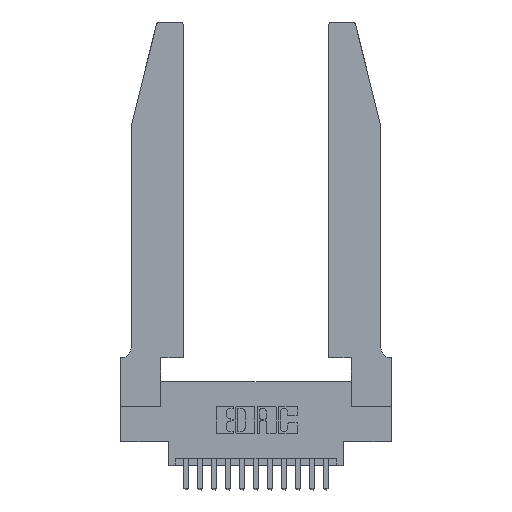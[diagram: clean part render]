
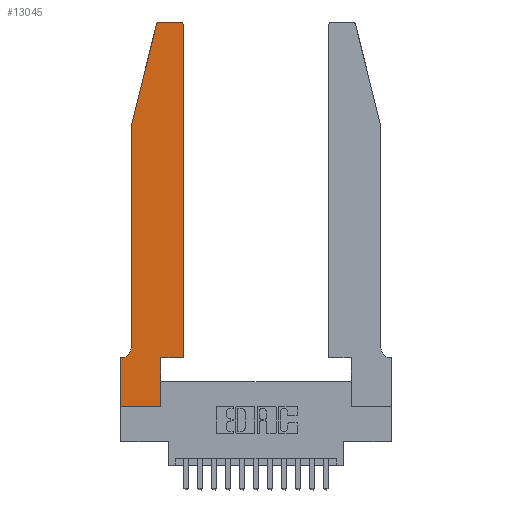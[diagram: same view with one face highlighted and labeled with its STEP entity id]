
A CAD part, top view. The second image highlights one B-rep face of the part: STEP entity #13045.
In plain terms, the highlighted planar face has unit normal (0, 0, 1).
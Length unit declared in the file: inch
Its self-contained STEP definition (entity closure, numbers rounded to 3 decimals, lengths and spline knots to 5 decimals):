
#377 = CARTESIAN_POINT ( 'NONE',  ( 0.0055, 0.35, 0.37 ) ) ;
#400 = EDGE_CURVE ( 'NONE', #11170, #15418, #11970, .T. ) ;
#570 = DIRECTION ( 'NONE',  ( 0., 0., -1. ) ) ;
#1208 = CARTESIAN_POINT ( 'NONE',  ( 0.0755, 0.35, 0.37 ) ) ;
#1275 = EDGE_LOOP ( 'NONE', ( #4739, #13195, #8741, #8817, #12159, #3597, #8021, #15969, #4738, #7466, #9636, #4335 ) ) ;
#1544 = VERTEX_POINT ( 'NONE', #4493 ) ;
#1551 = CIRCLE ( 'NONE', #7059, 0.03 ) ;
#1685 = LINE ( 'NONE', #3859, #11786 ) ;
#1721 = CARTESIAN_POINT ( 'NONE',  ( 0.4505, 2.72, 0.37 ) ) ;
#1910 = LINE ( 'NONE', #7632, #5176 ) ;
#1978 = FACE_OUTER_BOUND ( 'NONE', #1275, .T. ) ;
#2134 = DIRECTION ( 'NONE',  ( -0.239, -0.971, 0. ) ) ;
#2139 = VERTEX_POINT ( 'NONE', #1721 ) ;
#2272 = VECTOR ( 'NONE', #16141, 39.37008 ) ;
#2835 = VERTEX_POINT ( 'NONE', #8503 ) ;
#2952 = DIRECTION ( 'NONE',  ( 0., -1., 0. ) ) ;
#3266 = CIRCLE ( 'NONE', #13099, 0.03 ) ;
#3464 = EDGE_CURVE ( 'NONE', #15039, #14809, #10603, .T. ) ;
#3597 = ORIENTED_EDGE ( 'NONE', *, *, #17119, .T. ) ;
#3839 = CARTESIAN_POINT ( 'NONE',  ( 0.284, 2.75, 0.37 ) ) ;
#3859 = CARTESIAN_POINT ( 'NONE',  ( 0.4505, 0.35, 0.37 ) ) ;
#4257 = AXIS2_PLACEMENT_3D ( 'NONE', #11421, #4598, #14184 ) ;
#4277 = VECTOR ( 'NONE', #15594, 39.37008 ) ;
#4335 = ORIENTED_EDGE ( 'NONE', *, *, #13483, .T. ) ;
#4493 = CARTESIAN_POINT ( 'NONE',  ( 0.25487, 2.72718, 0.37 ) ) ;
#4598 = DIRECTION ( 'NONE',  ( 0., 0., 1. ) ) ;
#4665 = EDGE_CURVE ( 'NONE', #2835, #5376, #10775, .T. ) ;
#4738 = ORIENTED_EDGE ( 'NONE', *, *, #400, .T. ) ;
#4739 = ORIENTED_EDGE ( 'NONE', *, *, #4665, .T. ) ;
#4741 = EDGE_CURVE ( 'NONE', #1544, #4983, #10352, .T. ) ;
#4758 = VERTEX_POINT ( 'NONE', #17173 ) ;
#4861 = CARTESIAN_POINT ( 'NONE',  ( 0.0755, 2., 0.37 ) ) ;
#4910 = DIRECTION ( 'NONE',  ( 0., 1., 0. ) ) ;
#4983 = VERTEX_POINT ( 'NONE', #9564 ) ;
#5176 = VECTOR ( 'NONE', #4910, 39.37008 ) ;
#5329 = CARTESIAN_POINT ( 'NONE',  ( 0.4205, 2.72, 0.37 ) ) ;
#5376 = VERTEX_POINT ( 'NONE', #3839 ) ;
#5891 = CARTESIAN_POINT ( 'NONE',  ( 0.2865, 0., 0.37 ) ) ;
#6089 = CARTESIAN_POINT ( 'NONE',  ( 0.2865, 0.35, 0.37 ) ) ;
#6273 = LINE ( 'NONE', #1208, #16716 ) ;
#6515 = EDGE_CURVE ( 'NONE', #15418, #10537, #1685, .T. ) ;
#6654 = CARTESIAN_POINT ( 'NONE',  ( 0.0755, 0.42, 0.37 ) ) ;
#6718 = DIRECTION ( 'NONE',  ( 1., 0., 0. ) ) ;
#6878 = DIRECTION ( 'NONE',  ( 0., 1., 0. ) ) ;
#7059 = AXIS2_PLACEMENT_3D ( 'NONE', #7509, #17018, #8874 ) ;
#7325 = VECTOR ( 'NONE', #2952, 39.37008 ) ;
#7466 = ORIENTED_EDGE ( 'NONE', *, *, #6515, .T. ) ;
#7509 = CARTESIAN_POINT ( 'NONE',  ( 0.284, 2.72, 0.37 ) ) ;
#7632 = CARTESIAN_POINT ( 'NONE',  ( 0.4505, 0.35, 0.37 ) ) ;
#8021 = ORIENTED_EDGE ( 'NONE', *, *, #9525, .T. ) ;
#8471 = CARTESIAN_POINT ( 'NONE',  ( 0.0755, 2., 0.37 ) ) ;
#8503 = CARTESIAN_POINT ( 'NONE',  ( 0.4205, 2.75, 0.37 ) ) ;
#8701 = PLANE ( 'NONE',  #4257 ) ;
#8741 = ORIENTED_EDGE ( 'NONE', *, *, #4741, .T. ) ;
#8817 = ORIENTED_EDGE ( 'NONE', *, *, #9351, .T. ) ;
#8874 = DIRECTION ( 'NONE',  ( 1., 0., 0. ) ) ;
#8885 = CARTESIAN_POINT ( 'NONE',  ( 0.0055, 0.42, 0.37 ) ) ;
#8993 = EDGE_CURVE ( 'NONE', #10537, #2139, #1910, .T. ) ;
#9351 = EDGE_CURVE ( 'NONE', #4983, #15039, #11357, .T. ) ;
#9525 = EDGE_CURVE ( 'NONE', #13062, #4758, #15203, .T. ) ;
#9564 = CARTESIAN_POINT ( 'NONE',  ( 0.0755, 2., 0.37 ) ) ;
#9636 = ORIENTED_EDGE ( 'NONE', *, *, #8993, .T. ) ;
#10256 = DIRECTION ( 'NONE',  ( -1., 0., 0. ) ) ;
#10352 = LINE ( 'NONE', #4861, #16721 ) ;
#10537 = VERTEX_POINT ( 'NONE', #13908 ) ;
#10603 = CIRCLE ( 'NONE', #11149, 0.07 ) ;
#10705 = DIRECTION ( 'NONE',  ( 1., 0., 0. ) ) ;
#10775 = LINE ( 'NONE', #11626, #13975 ) ;
#10837 = EDGE_CURVE ( 'NONE', #4758, #11170, #17282, .T. ) ;
#10852 = DIRECTION ( 'NONE',  ( -1., 0., 0. ) ) ;
#11149 = AXIS2_PLACEMENT_3D ( 'NONE', #8885, #570, #10256 ) ;
#11170 = VERTEX_POINT ( 'NONE', #5891 ) ;
#11357 = LINE ( 'NONE', #8471, #7325 ) ;
#11421 = CARTESIAN_POINT ( 'NONE',  ( 0., 0.35, 0.37 ) ) ;
#11626 = CARTESIAN_POINT ( 'NONE',  ( 0.2605, 2.75, 0.37 ) ) ;
#11786 = VECTOR ( 'NONE', #10705, 39.37008 ) ;
#11970 = LINE ( 'NONE', #12056, #15606 ) ;
#12025 = CARTESIAN_POINT ( 'NONE',  ( 0., 0., 0.37 ) ) ;
#12056 = CARTESIAN_POINT ( 'NONE',  ( 0.2865, 0.35, 0.37 ) ) ;
#12159 = ORIENTED_EDGE ( 'NONE', *, *, #3464, .T. ) ;
#13004 = DIRECTION ( 'NONE',  ( -1., 0., 0. ) ) ;
#13045 = ADVANCED_FACE ( 'NONE', ( #1978 ), #8701, .T. ) ;
#13062 = VERTEX_POINT ( 'NONE', #15544 ) ;
#13099 = AXIS2_PLACEMENT_3D ( 'NONE', #5329, #14875, #6718 ) ;
#13106 = EDGE_CURVE ( 'NONE', #5376, #1544, #1551, .T. ) ;
#13195 = ORIENTED_EDGE ( 'NONE', *, *, #13106, .T. ) ;
#13483 = EDGE_CURVE ( 'NONE', #2139, #2835, #3266, .T. ) ;
#13908 = CARTESIAN_POINT ( 'NONE',  ( 0.4505, 0.35, 0.37 ) ) ;
#13975 = VECTOR ( 'NONE', #13004, 39.37008 ) ;
#14184 = DIRECTION ( 'NONE',  ( 1., 0., 0. ) ) ;
#14235 = CARTESIAN_POINT ( 'NONE',  ( 0., 0., 0.37 ) ) ;
#14809 = VERTEX_POINT ( 'NONE', #377 ) ;
#14875 = DIRECTION ( 'NONE',  ( 0., 0., 1. ) ) ;
#15039 = VERTEX_POINT ( 'NONE', #6654 ) ;
#15203 = LINE ( 'NONE', #14235, #4277 ) ;
#15418 = VERTEX_POINT ( 'NONE', #6089 ) ;
#15544 = CARTESIAN_POINT ( 'NONE',  ( 0., 0.35, 0.37 ) ) ;
#15594 = DIRECTION ( 'NONE',  ( 0., -1., 0. ) ) ;
#15606 = VECTOR ( 'NONE', #6878, 39.37008 ) ;
#15969 = ORIENTED_EDGE ( 'NONE', *, *, #10837, .T. ) ;
#16141 = DIRECTION ( 'NONE',  ( 1., 0., 0. ) ) ;
#16716 = VECTOR ( 'NONE', #10852, 39.37008 ) ;
#16721 = VECTOR ( 'NONE', #2134, 39.37008 ) ;
#17018 = DIRECTION ( 'NONE',  ( 0., 0., 1. ) ) ;
#17119 = EDGE_CURVE ( 'NONE', #14809, #13062, #6273, .T. ) ;
#17173 = CARTESIAN_POINT ( 'NONE',  ( 0., 0., 0.37 ) ) ;
#17282 = LINE ( 'NONE', #12025, #2272 ) ;
